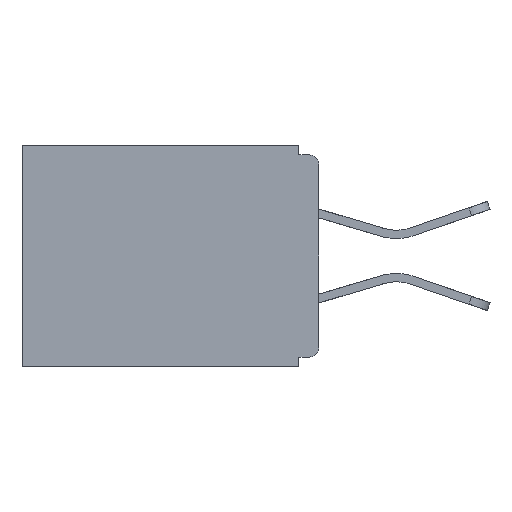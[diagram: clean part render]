
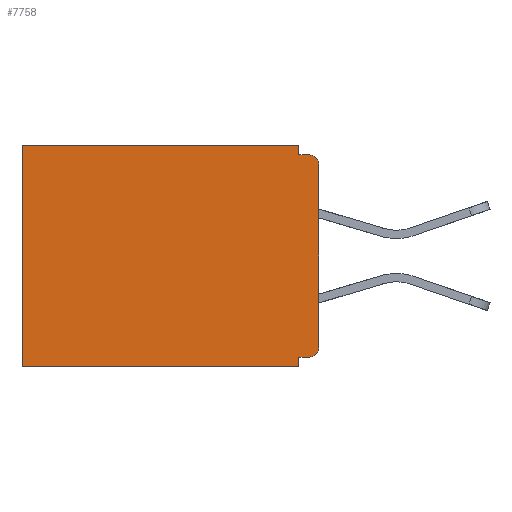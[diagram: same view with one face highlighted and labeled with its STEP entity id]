
A CAD part, left-side view. The second image highlights one B-rep face of the part: STEP entity #7758.
In plain terms, the highlighted planar face has unit normal (-1, 0, 0).
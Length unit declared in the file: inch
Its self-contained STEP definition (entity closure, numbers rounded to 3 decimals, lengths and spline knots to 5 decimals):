
#487 = DIRECTION ( 'NONE',  ( 0., 0., -1. ) ) ;
#554 = EDGE_CURVE ( 'NONE', #20893, #13459, #5147, .T. ) ;
#924 = EDGE_CURVE ( 'NONE', #18225, #8687, #5111, .T. ) ;
#1069 = VERTEX_POINT ( 'NONE', #20970 ) ;
#1186 = VECTOR ( 'NONE', #24785, 39.37008 ) ;
#1459 = PLANE ( 'NONE',  #21167 ) ;
#1590 = LINE ( 'NONE', #9365, #7221 ) ;
#1812 = CARTESIAN_POINT ( 'NONE',  ( 0.298, 0., -0.03 ) ) ;
#1925 = CARTESIAN_POINT ( 'NONE',  ( 0.298, 0.46, -0.343 ) ) ;
#2310 = CARTESIAN_POINT ( 'NONE',  ( 0.298, 0.46, 0. ) ) ;
#2484 = VECTOR ( 'NONE', #12510, 39.37008 ) ;
#4155 = EDGE_LOOP ( 'NONE', ( #15931, #8086, #6405, #24668, #27367, #13986, #20064, #20687, #18672, #24360 ) ) ;
#4288 = CARTESIAN_POINT ( 'NONE',  ( 0.298, 0.031, -0.343 ) ) ;
#4344 = VERTEX_POINT ( 'NONE', #1812 ) ;
#4482 = LINE ( 'NONE', #26910, #22810 ) ;
#5111 = LINE ( 'NONE', #17397, #19137 ) ;
#5147 = LINE ( 'NONE', #6736, #2484 ) ;
#5544 = EDGE_CURVE ( 'NONE', #1069, #26857, #4482, .T. ) ;
#6405 = ORIENTED_EDGE ( 'NONE', *, *, #924, .F. ) ;
#6736 = CARTESIAN_POINT ( 'NONE',  ( 0.298, 0., -0.328 ) ) ;
#6822 = FACE_OUTER_BOUND ( 'NONE', #4155, .T. ) ;
#7107 = CARTESIAN_POINT ( 'NONE',  ( 0.298, 0.015, -0.313 ) ) ;
#7221 = VECTOR ( 'NONE', #7300, 39.37008 ) ;
#7300 = DIRECTION ( 'NONE',  ( 0., 0., -1. ) ) ;
#7408 = AXIS2_PLACEMENT_3D ( 'NONE', #7107, #26365, #11472 ) ;
#7758 = ADVANCED_FACE ( 'NONE', ( #6822 ), #1459, .F. ) ;
#8005 = VECTOR ( 'NONE', #15686, 39.37008 ) ;
#8086 = ORIENTED_EDGE ( 'NONE', *, *, #25697, .F. ) ;
#8687 = VERTEX_POINT ( 'NONE', #16011 ) ;
#9365 = CARTESIAN_POINT ( 'NONE',  ( 0.298, 0., 0. ) ) ;
#9421 = CIRCLE ( 'NONE', #7408, 0.015 ) ;
#9613 = EDGE_CURVE ( 'NONE', #20893, #26727, #9421, .T. ) ;
#9720 = EDGE_CURVE ( 'NONE', #22180, #26857, #12412, .T. ) ;
#10858 = LINE ( 'NONE', #23667, #12184 ) ;
#10909 = DIRECTION ( 'NONE',  ( 0., -1., 0. ) ) ;
#11472 = DIRECTION ( 'NONE',  ( 0., 0., -1. ) ) ;
#11949 = CARTESIAN_POINT ( 'NONE',  ( 0.298, 0., -0.313 ) ) ;
#12113 = CARTESIAN_POINT ( 'NONE',  ( 0.298, 0., 0. ) ) ;
#12184 = VECTOR ( 'NONE', #10909, 39.37008 ) ;
#12412 = LINE ( 'NONE', #24044, #25716 ) ;
#12510 = DIRECTION ( 'NONE',  ( 0., 1., 0. ) ) ;
#12786 = CARTESIAN_POINT ( 'NONE',  ( 0.298, 0.015, -0.015 ) ) ;
#13235 = EDGE_CURVE ( 'NONE', #4344, #13291, #18871, .T. ) ;
#13291 = VERTEX_POINT ( 'NONE', #12786 ) ;
#13411 = CARTESIAN_POINT ( 'NONE',  ( 0.298, 0.031, -0.328 ) ) ;
#13428 = DIRECTION ( 'NONE',  ( 0., 0., -1. ) ) ;
#13459 = VERTEX_POINT ( 'NONE', #13411 ) ;
#13955 = DIRECTION ( 'NONE',  ( 0., 1., 0. ) ) ;
#13986 = ORIENTED_EDGE ( 'NONE', *, *, #5544, .F. ) ;
#15402 = EDGE_CURVE ( 'NONE', #4344, #26727, #1590, .T. ) ;
#15435 = AXIS2_PLACEMENT_3D ( 'NONE', #21314, #23398, #27209 ) ;
#15686 = DIRECTION ( 'NONE',  ( 0., 0., -1. ) ) ;
#15931 = ORIENTED_EDGE ( 'NONE', *, *, #13235, .T. ) ;
#16011 = CARTESIAN_POINT ( 'NONE',  ( 0.298, 0.031, -0.015 ) ) ;
#16142 = CARTESIAN_POINT ( 'NONE',  ( 0.298, 0.015, -0.328 ) ) ;
#17397 = CARTESIAN_POINT ( 'NONE',  ( 0.298, 0.031, -0.343 ) ) ;
#17773 = CARTESIAN_POINT ( 'NONE',  ( 0.298, 0.031, 0. ) ) ;
#18225 = VERTEX_POINT ( 'NONE', #17773 ) ;
#18672 = ORIENTED_EDGE ( 'NONE', *, *, #9613, .T. ) ;
#18871 = CIRCLE ( 'NONE', #15435, 0.015 ) ;
#19137 = VECTOR ( 'NONE', #487, 39.37008 ) ;
#20064 = ORIENTED_EDGE ( 'NONE', *, *, #22954, .F. ) ;
#20556 = DIRECTION ( 'NONE',  ( 1., 0., 0. ) ) ;
#20687 = ORIENTED_EDGE ( 'NONE', *, *, #554, .F. ) ;
#20893 = VERTEX_POINT ( 'NONE', #16142 ) ;
#20970 = CARTESIAN_POINT ( 'NONE',  ( 0.298, 0.031, -0.343 ) ) ;
#21058 = LINE ( 'NONE', #4288, #8005 ) ;
#21167 = AXIS2_PLACEMENT_3D ( 'NONE', #26825, #20556, #22650 ) ;
#21170 = EDGE_CURVE ( 'NONE', #18225, #22180, #23806, .T. ) ;
#21314 = CARTESIAN_POINT ( 'NONE',  ( 0.298, 0.015, -0.03 ) ) ;
#22180 = VERTEX_POINT ( 'NONE', #2310 ) ;
#22650 = DIRECTION ( 'NONE',  ( 0., 0., -1. ) ) ;
#22810 = VECTOR ( 'NONE', #13955, 39.37008 ) ;
#22954 = EDGE_CURVE ( 'NONE', #13459, #1069, #21058, .T. ) ;
#23398 = DIRECTION ( 'NONE',  ( -1., 0., 0. ) ) ;
#23667 = CARTESIAN_POINT ( 'NONE',  ( 0.298, 0., -0.015 ) ) ;
#23806 = LINE ( 'NONE', #12113, #1186 ) ;
#24044 = CARTESIAN_POINT ( 'NONE',  ( 0.298, 0.46, 0. ) ) ;
#24360 = ORIENTED_EDGE ( 'NONE', *, *, #15402, .F. ) ;
#24668 = ORIENTED_EDGE ( 'NONE', *, *, #21170, .T. ) ;
#24785 = DIRECTION ( 'NONE',  ( 0., 1., 0. ) ) ;
#25697 = EDGE_CURVE ( 'NONE', #8687, #13291, #10858, .T. ) ;
#25716 = VECTOR ( 'NONE', #13428, 39.37008 ) ;
#26365 = DIRECTION ( 'NONE',  ( -1., 0., 0. ) ) ;
#26727 = VERTEX_POINT ( 'NONE', #11949 ) ;
#26825 = CARTESIAN_POINT ( 'NONE',  ( 0.298, 0., 0. ) ) ;
#26857 = VERTEX_POINT ( 'NONE', #1925 ) ;
#26910 = CARTESIAN_POINT ( 'NONE',  ( 0.298, 0., -0.343 ) ) ;
#27209 = DIRECTION ( 'NONE',  ( 0., 0., -1. ) ) ;
#27367 = ORIENTED_EDGE ( 'NONE', *, *, #9720, .T. ) ;
